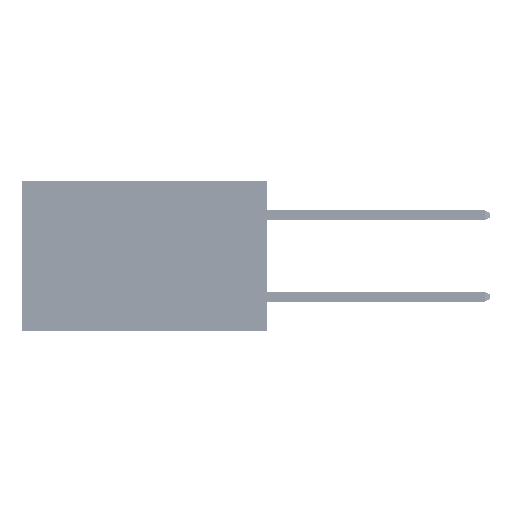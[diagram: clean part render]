
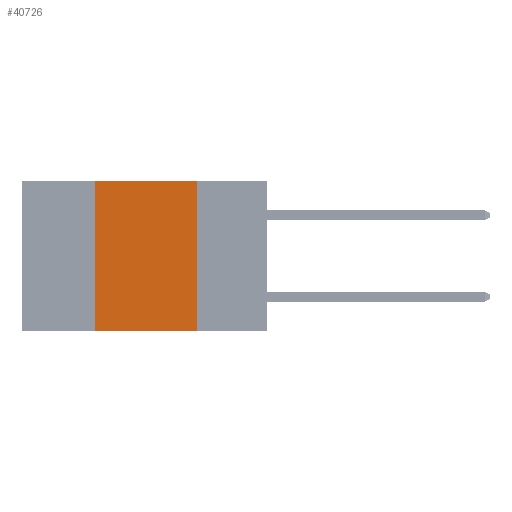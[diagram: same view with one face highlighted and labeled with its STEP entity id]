
A CAD part, left-side view. The second image highlights one B-rep face of the part: STEP entity #40726.
In plain terms, the highlighted planar face has unit normal (-1, 0, 0).
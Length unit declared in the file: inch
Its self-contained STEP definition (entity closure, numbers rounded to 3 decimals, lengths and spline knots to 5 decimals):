
#332 = LINE ( 'NONE', #30422, #20776 ) ;
#1448 = CARTESIAN_POINT ( 'NONE',  ( 0., 0.42, 0. ) ) ;
#5098 = ORIENTED_EDGE ( 'NONE', *, *, #8294, .F. ) ;
#8294 = EDGE_CURVE ( 'NONE', #22978, #41781, #332, .T. ) ;
#10911 = EDGE_CURVE ( 'NONE', #25438, #25087, #37988, .T. ) ;
#11808 = CARTESIAN_POINT ( 'NONE',  ( 0., 0.17, -0.37 ) ) ;
#15286 = CARTESIAN_POINT ( 'NONE',  ( 0., 0.17, 0. ) ) ;
#17854 = DIRECTION ( 'NONE',  ( 0., 0., 1. ) ) ;
#18410 = ORIENTED_EDGE ( 'NONE', *, *, #10911, .F. ) ;
#20776 = VECTOR ( 'NONE', #46009, 39.37008 ) ;
#21168 = DIRECTION ( 'NONE',  ( 0., -1., 0. ) ) ;
#22557 = CARTESIAN_POINT ( 'NONE',  ( 0., 0.42, -0.37 ) ) ;
#22978 = VERTEX_POINT ( 'NONE', #15286 ) ;
#23560 = DIRECTION ( 'NONE',  ( 0., -1., 0. ) ) ;
#23794 = DIRECTION ( 'NONE',  ( 0., 0., -1. ) ) ;
#24346 = LINE ( 'NONE', #31855, #45760 ) ;
#25087 = VERTEX_POINT ( 'NONE', #51814 ) ;
#25438 = VERTEX_POINT ( 'NONE', #22557 ) ;
#28916 = EDGE_LOOP ( 'NONE', ( #5098, #51417, #18410, #49871 ) ) ;
#29081 = VECTOR ( 'NONE', #17854, 39.37008 ) ;
#30147 = AXIS2_PLACEMENT_3D ( 'NONE', #47933, #47673, #23794 ) ;
#30422 = CARTESIAN_POINT ( 'NONE',  ( 0., 0.17, 0. ) ) ;
#31034 = FACE_OUTER_BOUND ( 'NONE', #28916, .T. ) ;
#31855 = CARTESIAN_POINT ( 'NONE',  ( 0., 0.6, 0. ) ) ;
#34037 = LINE ( 'NONE', #37523, #40638 ) ;
#36056 = EDGE_CURVE ( 'NONE', #25087, #22978, #24346, .T. ) ;
#36395 = EDGE_CURVE ( 'NONE', #25438, #41781, #34037, .T. ) ;
#37523 = CARTESIAN_POINT ( 'NONE',  ( 0., 0.6, -0.37 ) ) ;
#37988 = LINE ( 'NONE', #1448, #29081 ) ;
#40638 = VECTOR ( 'NONE', #21168, 39.37008 ) ;
#40726 = ADVANCED_FACE ( 'NONE', ( #31034 ), #43381, .F. ) ;
#41781 = VERTEX_POINT ( 'NONE', #11808 ) ;
#43381 = PLANE ( 'NONE',  #30147 ) ;
#45760 = VECTOR ( 'NONE', #23560, 39.37008 ) ;
#46009 = DIRECTION ( 'NONE',  ( 0., 0., -1. ) ) ;
#47673 = DIRECTION ( 'NONE',  ( 1., 0., 0. ) ) ;
#47933 = CARTESIAN_POINT ( 'NONE',  ( 0., 0.6, 0. ) ) ;
#49871 = ORIENTED_EDGE ( 'NONE', *, *, #36395, .T. ) ;
#51417 = ORIENTED_EDGE ( 'NONE', *, *, #36056, .F. ) ;
#51814 = CARTESIAN_POINT ( 'NONE',  ( 0., 0.42, 0. ) ) ;
